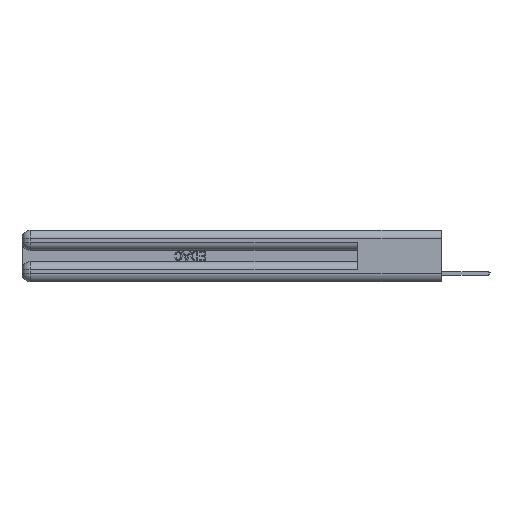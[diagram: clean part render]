
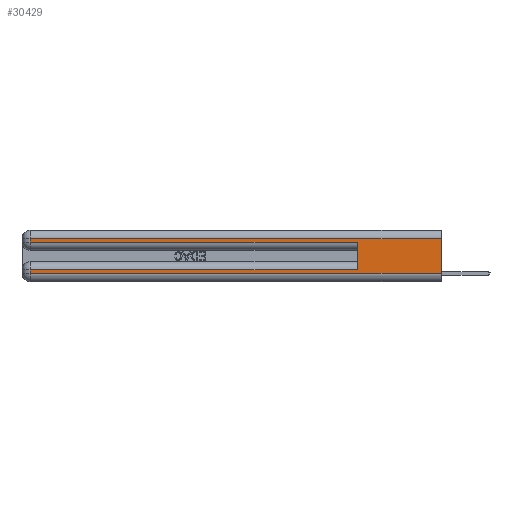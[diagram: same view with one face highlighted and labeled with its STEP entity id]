
A CAD part, left-side view. The second image highlights one B-rep face of the part: STEP entity #30429.
In plain terms, the highlighted planar face has unit normal (-1, 0, 0).
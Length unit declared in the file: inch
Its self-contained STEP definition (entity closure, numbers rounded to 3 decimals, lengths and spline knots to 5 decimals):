
#1386 = ORIENTED_EDGE ( 'NONE', *, *, #33027, .T. ) ;
#2485 = EDGE_CURVE ( 'NONE', #12525, #8493, #5876, .T. ) ;
#2948 = CARTESIAN_POINT ( 'NONE',  ( 0., 0., 0.31 ) ) ;
#3000 = EDGE_CURVE ( 'NONE', #12525, #26868, #27930, .T. ) ;
#3782 = LINE ( 'NONE', #14324, #24009 ) ;
#3923 = DIRECTION ( 'NONE',  ( 0., 0., -1. ) ) ;
#5054 = VERTEX_POINT ( 'NONE', #29416 ) ;
#5582 = VECTOR ( 'NONE', #15634, 39.37008 ) ;
#5876 = LINE ( 'NONE', #2948, #11371 ) ;
#6127 = ORIENTED_EDGE ( 'NONE', *, *, #26797, .T. ) ;
#7462 = CARTESIAN_POINT ( 'NONE',  ( 0., 2.94, 0.37 ) ) ;
#7793 = VECTOR ( 'NONE', #29755, 39.37008 ) ;
#8493 = VERTEX_POINT ( 'NONE', #9531 ) ;
#8933 = VECTOR ( 'NONE', #17750, 39.37008 ) ;
#9098 = VECTOR ( 'NONE', #17490, 39.37008 ) ;
#9531 = CARTESIAN_POINT ( 'NONE',  ( 0., 2.94, 0.31 ) ) ;
#9772 = CARTESIAN_POINT ( 'NONE',  ( 0., 0., 0.085 ) ) ;
#10386 = EDGE_CURVE ( 'NONE', #8493, #30726, #20513, .T. ) ;
#10706 = DIRECTION ( 'NONE',  ( 0., 1., 0. ) ) ;
#11371 = VECTOR ( 'NONE', #10706, 39.37008 ) ;
#12473 = EDGE_CURVE ( 'NONE', #14766, #28831, #15138, .T. ) ;
#12479 = LINE ( 'NONE', #7462, #9098 ) ;
#12525 = VERTEX_POINT ( 'NONE', #33458 ) ;
#12805 = ORIENTED_EDGE ( 'NONE', *, *, #3000, .F. ) ;
#13156 = CARTESIAN_POINT ( 'NONE',  ( 0., 0.6, 0.085 ) ) ;
#13539 = DIRECTION ( 'NONE',  ( 1., 0., 0. ) ) ;
#13721 = CARTESIAN_POINT ( 'NONE',  ( 0., 0., 0.37 ) ) ;
#14301 = CARTESIAN_POINT ( 'NONE',  ( 0., 0., 0.37 ) ) ;
#14324 = CARTESIAN_POINT ( 'NONE',  ( 0., 0., 0.06 ) ) ;
#14766 = VERTEX_POINT ( 'NONE', #13156 ) ;
#15138 = LINE ( 'NONE', #23086, #29356 ) ;
#15634 = DIRECTION ( 'NONE',  ( 0., 1., 0. ) ) ;
#16680 = CARTESIAN_POINT ( 'NONE',  ( 0., 0.6, 0.285 ) ) ;
#17490 = DIRECTION ( 'NONE',  ( 0., 0., -1. ) ) ;
#17750 = DIRECTION ( 'NONE',  ( 0., 0., -1. ) ) ;
#17896 = VERTEX_POINT ( 'NONE', #20520 ) ;
#19325 = DIRECTION ( 'NONE',  ( 0., -1., 0. ) ) ;
#20513 = LINE ( 'NONE', #25874, #8933 ) ;
#20520 = CARTESIAN_POINT ( 'NONE',  ( 0., 2.94, 0.085 ) ) ;
#20649 = LINE ( 'NONE', #9772, #5582 ) ;
#21379 = ORIENTED_EDGE ( 'NONE', *, *, #12473, .F. ) ;
#22886 = AXIS2_PLACEMENT_3D ( 'NONE', #13721, #13539, #26671 ) ;
#23086 = CARTESIAN_POINT ( 'NONE',  ( 0., 0.6, 0.145 ) ) ;
#24009 = VECTOR ( 'NONE', #19325, 39.37008 ) ;
#24425 = FACE_OUTER_BOUND ( 'NONE', #33370, .T. ) ;
#24521 = ORIENTED_EDGE ( 'NONE', *, *, #10386, .T. ) ;
#25874 = CARTESIAN_POINT ( 'NONE',  ( 0., 2.94, 0.37 ) ) ;
#26604 = ORIENTED_EDGE ( 'NONE', *, *, #32447, .T. ) ;
#26671 = DIRECTION ( 'NONE',  ( 0., 0., -1. ) ) ;
#26797 = EDGE_CURVE ( 'NONE', #14766, #17896, #20649, .T. ) ;
#26868 = VERTEX_POINT ( 'NONE', #31702 ) ;
#26987 = LINE ( 'NONE', #27318, #7793 ) ;
#27318 = CARTESIAN_POINT ( 'NONE',  ( 0., 0., 0.285 ) ) ;
#27487 = EDGE_CURVE ( 'NONE', #30726, #28831, #26987, .T. ) ;
#27930 = LINE ( 'NONE', #14301, #33478 ) ;
#27935 = DIRECTION ( 'NONE',  ( 0., 0., 1. ) ) ;
#28831 = VERTEX_POINT ( 'NONE', #16680 ) ;
#29356 = VECTOR ( 'NONE', #27935, 39.37008 ) ;
#29416 = CARTESIAN_POINT ( 'NONE',  ( 0., 2.94, 0.06 ) ) ;
#29755 = DIRECTION ( 'NONE',  ( 0., -1., 0. ) ) ;
#29953 = PLANE ( 'NONE',  #22886 ) ;
#30429 = ADVANCED_FACE ( 'NONE', ( #24425 ), #29953, .F. ) ;
#30726 = VERTEX_POINT ( 'NONE', #31307 ) ;
#31307 = CARTESIAN_POINT ( 'NONE',  ( 0., 2.94, 0.285 ) ) ;
#31702 = CARTESIAN_POINT ( 'NONE',  ( 0., 0., 0.06 ) ) ;
#32143 = ORIENTED_EDGE ( 'NONE', *, *, #27487, .T. ) ;
#32447 = EDGE_CURVE ( 'NONE', #17896, #5054, #12479, .T. ) ;
#32742 = ORIENTED_EDGE ( 'NONE', *, *, #2485, .T. ) ;
#33027 = EDGE_CURVE ( 'NONE', #5054, #26868, #3782, .T. ) ;
#33370 = EDGE_LOOP ( 'NONE', ( #12805, #32742, #24521, #32143, #21379, #6127, #26604, #1386 ) ) ;
#33458 = CARTESIAN_POINT ( 'NONE',  ( 0., 0., 0.31 ) ) ;
#33478 = VECTOR ( 'NONE', #3923, 39.37008 ) ;
